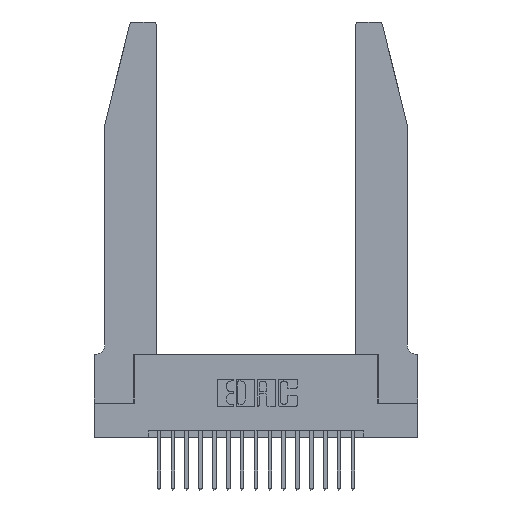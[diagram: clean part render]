
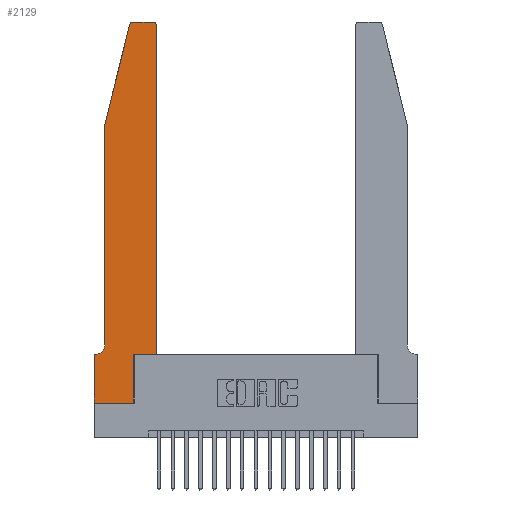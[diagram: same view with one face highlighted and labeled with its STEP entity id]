
A CAD part, top view. The second image highlights one B-rep face of the part: STEP entity #2129.
In plain terms, the highlighted planar face has unit normal (0, 0, 1).
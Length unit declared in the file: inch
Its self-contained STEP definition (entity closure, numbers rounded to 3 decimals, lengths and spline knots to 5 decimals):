
#8 = CARTESIAN_POINT ( 'NONE',  ( 0.4205, 2.72, 0.37 ) ) ;
#345 = CARTESIAN_POINT ( 'NONE',  ( 0., 0., 0.37 ) ) ;
#613 = EDGE_CURVE ( 'NONE', #12728, #14184, #3312, .T. ) ;
#794 = EDGE_LOOP ( 'NONE', ( #19280, #2100, #8696, #6594, #17801, #17340, #1324, #6926, #3165, #8301, #17634, #5933 ) ) ;
#826 = LINE ( 'NONE', #12022, #13554 ) ;
#925 = CARTESIAN_POINT ( 'NONE',  ( 0.0755, 0.42, 0.37 ) ) ;
#1324 = ORIENTED_EDGE ( 'NONE', *, *, #9957, .T. ) ;
#1944 = DIRECTION ( 'NONE',  ( 0., 0., 1. ) ) ;
#2048 = CARTESIAN_POINT ( 'NONE',  ( 0.4505, 0.35, 0.37 ) ) ;
#2067 = VERTEX_POINT ( 'NONE', #16862 ) ;
#2100 = ORIENTED_EDGE ( 'NONE', *, *, #2959, .T. ) ;
#2108 = VECTOR ( 'NONE', #14891, 39.37008 ) ;
#2129 = ADVANCED_FACE ( 'NONE', ( #15678 ), #13830, .T. ) ;
#2959 = EDGE_CURVE ( 'NONE', #10581, #12728, #12000, .T. ) ;
#2996 = LINE ( 'NONE', #9786, #16154 ) ;
#3089 = CARTESIAN_POINT ( 'NONE',  ( 0., 0., 0.37 ) ) ;
#3123 = EDGE_CURVE ( 'NONE', #3171, #10581, #13462, .T. ) ;
#3165 = ORIENTED_EDGE ( 'NONE', *, *, #9988, .T. ) ;
#3171 = VERTEX_POINT ( 'NONE', #14517 ) ;
#3255 = DIRECTION ( 'NONE',  ( 0., -1., 0. ) ) ;
#3312 = LINE ( 'NONE', #12470, #15259 ) ;
#3323 = CARTESIAN_POINT ( 'NONE',  ( 0., 0., 0.37 ) ) ;
#3404 = EDGE_CURVE ( 'NONE', #16867, #2067, #5611, .T. ) ;
#3545 = CARTESIAN_POINT ( 'NONE',  ( 0.284, 2.75, 0.37 ) ) ;
#3850 = CARTESIAN_POINT ( 'NONE',  ( 0.0755, 0.35, 0.37 ) ) ;
#4050 = DIRECTION ( 'NONE',  ( 1., 0., 0. ) ) ;
#4141 = DIRECTION ( 'NONE',  ( 1., 0., 0. ) ) ;
#4658 = CARTESIAN_POINT ( 'NONE',  ( 0.2865, 0., 0.37 ) ) ;
#4802 = DIRECTION ( 'NONE',  ( -1., 0., 0. ) ) ;
#5611 = CIRCLE ( 'NONE', #13747, 0.07 ) ;
#5754 = AXIS2_PLACEMENT_3D ( 'NONE', #13619, #12246, #19855 ) ;
#5933 = ORIENTED_EDGE ( 'NONE', *, *, #14085, .T. ) ;
#6060 = LINE ( 'NONE', #11206, #17039 ) ;
#6063 = CARTESIAN_POINT ( 'NONE',  ( 0.2865, 0.35, 0.37 ) ) ;
#6169 = VERTEX_POINT ( 'NONE', #11761 ) ;
#6298 = DIRECTION ( 'NONE',  ( 0., 1., 0. ) ) ;
#6480 = VERTEX_POINT ( 'NONE', #4658 ) ;
#6594 = ORIENTED_EDGE ( 'NONE', *, *, #7748, .T. ) ;
#6926 = ORIENTED_EDGE ( 'NONE', *, *, #19671, .T. ) ;
#7024 = CARTESIAN_POINT ( 'NONE',  ( 0.4505, 0.35, 0.37 ) ) ;
#7109 = EDGE_CURVE ( 'NONE', #10446, #19162, #826, .T. ) ;
#7355 = CARTESIAN_POINT ( 'NONE',  ( 0.25487, 2.72718, 0.37 ) ) ;
#7748 = EDGE_CURVE ( 'NONE', #14184, #16867, #2996, .T. ) ;
#7845 = DIRECTION ( 'NONE',  ( 0., 0., 1. ) ) ;
#8177 = LINE ( 'NONE', #2048, #18933 ) ;
#8206 = AXIS2_PLACEMENT_3D ( 'NONE', #8, #7845, #14212 ) ;
#8296 = VERTEX_POINT ( 'NONE', #3089 ) ;
#8301 = ORIENTED_EDGE ( 'NONE', *, *, #7109, .T. ) ;
#8696 = ORIENTED_EDGE ( 'NONE', *, *, #613, .T. ) ;
#9786 = CARTESIAN_POINT ( 'NONE',  ( 0.0755, 2., 0.37 ) ) ;
#9957 = EDGE_CURVE ( 'NONE', #6169, #8296, #19208, .T. ) ;
#9962 = DIRECTION ( 'NONE',  ( 0., 1., 0. ) ) ;
#9988 = EDGE_CURVE ( 'NONE', #6480, #10446, #6060, .T. ) ;
#10400 = DIRECTION ( 'NONE',  ( 0., 0., -1. ) ) ;
#10446 = VERTEX_POINT ( 'NONE', #6063 ) ;
#10581 = VERTEX_POINT ( 'NONE', #3545 ) ;
#10937 = EDGE_CURVE ( 'NONE', #2067, #6169, #12665, .T. ) ;
#11006 = VECTOR ( 'NONE', #4802, 39.37008 ) ;
#11206 = CARTESIAN_POINT ( 'NONE',  ( 0.2865, 0.35, 0.37 ) ) ;
#11321 = DIRECTION ( 'NONE',  ( 1., 0., 0. ) ) ;
#11371 = EDGE_CURVE ( 'NONE', #19162, #18863, #8177, .T. ) ;
#11761 = CARTESIAN_POINT ( 'NONE',  ( 0., 0.35, 0.37 ) ) ;
#12000 = CIRCLE ( 'NONE', #19305, 0.03 ) ;
#12022 = CARTESIAN_POINT ( 'NONE',  ( 0.4505, 0.35, 0.37 ) ) ;
#12246 = DIRECTION ( 'NONE',  ( 0., 0., 1. ) ) ;
#12470 = CARTESIAN_POINT ( 'NONE',  ( 0.0755, 2., 0.37 ) ) ;
#12665 = LINE ( 'NONE', #3850, #2108 ) ;
#12728 = VERTEX_POINT ( 'NONE', #7355 ) ;
#13104 = DIRECTION ( 'NONE',  ( 0., -1., 0. ) ) ;
#13275 = DIRECTION ( 'NONE',  ( -1., 0., 0. ) ) ;
#13462 = LINE ( 'NONE', #17139, #11006 ) ;
#13554 = VECTOR ( 'NONE', #4141, 39.37008 ) ;
#13619 = CARTESIAN_POINT ( 'NONE',  ( 0., 0.35, 0.37 ) ) ;
#13747 = AXIS2_PLACEMENT_3D ( 'NONE', #19720, #10400, #13275 ) ;
#13830 = PLANE ( 'NONE',  #5754 ) ;
#14085 = EDGE_CURVE ( 'NONE', #18863, #3171, #19835, .T. ) ;
#14184 = VERTEX_POINT ( 'NONE', #18947 ) ;
#14212 = DIRECTION ( 'NONE',  ( 1., 0., 0. ) ) ;
#14517 = CARTESIAN_POINT ( 'NONE',  ( 0.4205, 2.75, 0.37 ) ) ;
#14772 = LINE ( 'NONE', #345, #20157 ) ;
#14891 = DIRECTION ( 'NONE',  ( -1., 0., 0. ) ) ;
#15259 = VECTOR ( 'NONE', #18490, 39.37008 ) ;
#15678 = FACE_OUTER_BOUND ( 'NONE', #794, .T. ) ;
#15820 = VECTOR ( 'NONE', #3255, 39.37008 ) ;
#16154 = VECTOR ( 'NONE', #13104, 39.37008 ) ;
#16862 = CARTESIAN_POINT ( 'NONE',  ( 0.0055, 0.35, 0.37 ) ) ;
#16867 = VERTEX_POINT ( 'NONE', #925 ) ;
#17039 = VECTOR ( 'NONE', #6298, 39.37008 ) ;
#17139 = CARTESIAN_POINT ( 'NONE',  ( 0.2605, 2.75, 0.37 ) ) ;
#17340 = ORIENTED_EDGE ( 'NONE', *, *, #10937, .T. ) ;
#17572 = CARTESIAN_POINT ( 'NONE',  ( 0.284, 2.72, 0.37 ) ) ;
#17634 = ORIENTED_EDGE ( 'NONE', *, *, #11371, .T. ) ;
#17801 = ORIENTED_EDGE ( 'NONE', *, *, #3404, .T. ) ;
#18490 = DIRECTION ( 'NONE',  ( -0.239, -0.971, 0. ) ) ;
#18837 = CARTESIAN_POINT ( 'NONE',  ( 0.4505, 2.72, 0.37 ) ) ;
#18863 = VERTEX_POINT ( 'NONE', #18837 ) ;
#18933 = VECTOR ( 'NONE', #9962, 39.37008 ) ;
#18947 = CARTESIAN_POINT ( 'NONE',  ( 0.0755, 2., 0.37 ) ) ;
#19162 = VERTEX_POINT ( 'NONE', #7024 ) ;
#19208 = LINE ( 'NONE', #3323, #15820 ) ;
#19280 = ORIENTED_EDGE ( 'NONE', *, *, #3123, .T. ) ;
#19305 = AXIS2_PLACEMENT_3D ( 'NONE', #17572, #1944, #4050 ) ;
#19671 = EDGE_CURVE ( 'NONE', #8296, #6480, #14772, .T. ) ;
#19720 = CARTESIAN_POINT ( 'NONE',  ( 0.0055, 0.42, 0.37 ) ) ;
#19835 = CIRCLE ( 'NONE', #8206, 0.03 ) ;
#19855 = DIRECTION ( 'NONE',  ( 1., 0., 0. ) ) ;
#20157 = VECTOR ( 'NONE', #11321, 39.37008 ) ;
